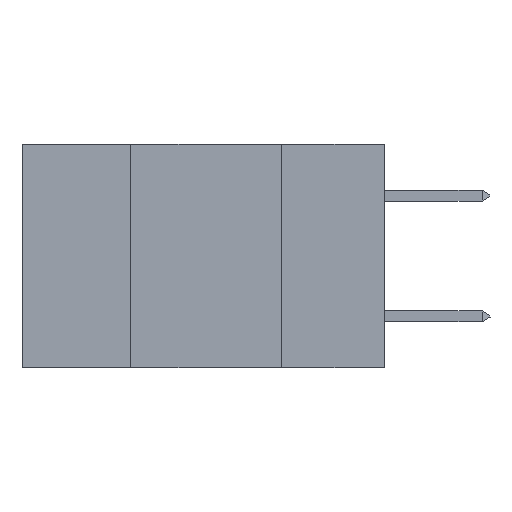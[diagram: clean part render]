
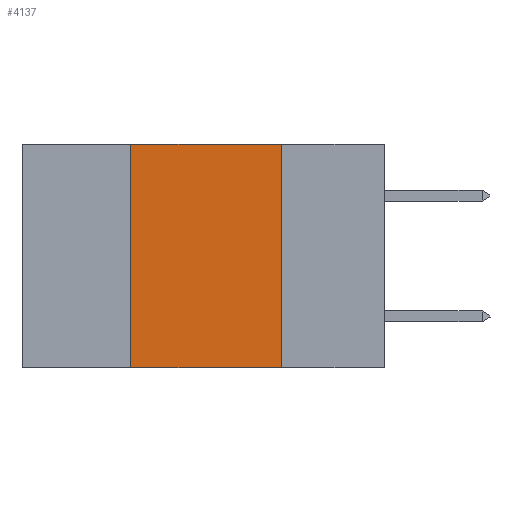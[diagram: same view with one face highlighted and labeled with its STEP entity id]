
A CAD part, left-side view. The second image highlights one B-rep face of the part: STEP entity #4137.
In plain terms, the highlighted planar face has unit normal (-1, 0, 0).
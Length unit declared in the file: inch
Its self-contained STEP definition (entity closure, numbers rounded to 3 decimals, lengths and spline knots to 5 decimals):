
#258 = DIRECTION ( 'NONE',  ( 0., 0., 1. ) ) ;
#322 = ORIENTED_EDGE ( 'NONE', *, *, #5474, .F. ) ;
#654 = CARTESIAN_POINT ( 'NONE',  ( 0., 0.42, 0. ) ) ;
#828 = CARTESIAN_POINT ( 'NONE',  ( 0., 0.17, 0. ) ) ;
#831 = VECTOR ( 'NONE', #3111, 39.37008 ) ;
#1708 = VERTEX_POINT ( 'NONE', #10347 ) ;
#1916 = LINE ( 'NONE', #5691, #11187 ) ;
#2489 = EDGE_CURVE ( 'NONE', #5838, #1708, #4367, .T. ) ;
#2636 = VECTOR ( 'NONE', #7221, 39.37008 ) ;
#3043 = CARTESIAN_POINT ( 'NONE',  ( 0., 0.17, 0. ) ) ;
#3111 = DIRECTION ( 'NONE',  ( 0., -1., 0. ) ) ;
#3341 = VECTOR ( 'NONE', #3395, 39.37008 ) ;
#3395 = DIRECTION ( 'NONE',  ( 0., 0., -1. ) ) ;
#3470 = LINE ( 'NONE', #828, #3341 ) ;
#4081 = ORIENTED_EDGE ( 'NONE', *, *, #5026, .F. ) ;
#4137 = ADVANCED_FACE ( 'NONE', ( #11146 ), #9200, .F. ) ;
#4367 = LINE ( 'NONE', #7265, #2636 ) ;
#4542 = EDGE_CURVE ( 'NONE', #10076, #1708, #3470, .T. ) ;
#4907 = EDGE_LOOP ( 'NONE', ( #11507, #4081, #322, #5097 ) ) ;
#5026 = EDGE_CURVE ( 'NONE', #5121, #10076, #9524, .T. ) ;
#5097 = ORIENTED_EDGE ( 'NONE', *, *, #2489, .T. ) ;
#5121 = VERTEX_POINT ( 'NONE', #654 ) ;
#5474 = EDGE_CURVE ( 'NONE', #5838, #5121, #1916, .T. ) ;
#5507 = CARTESIAN_POINT ( 'NONE',  ( 0., 0.42, -0.37 ) ) ;
#5691 = CARTESIAN_POINT ( 'NONE',  ( 0., 0.42, 0. ) ) ;
#5838 = VERTEX_POINT ( 'NONE', #5507 ) ;
#6012 = DIRECTION ( 'NONE',  ( 1., 0., 0. ) ) ;
#7221 = DIRECTION ( 'NONE',  ( 0., -1., 0. ) ) ;
#7265 = CARTESIAN_POINT ( 'NONE',  ( 0., 0.6, -0.37 ) ) ;
#7489 = CARTESIAN_POINT ( 'NONE',  ( 0., 0.6, 0. ) ) ;
#7505 = DIRECTION ( 'NONE',  ( 0., 0., -1. ) ) ;
#7724 = CARTESIAN_POINT ( 'NONE',  ( 0., 0.6, 0. ) ) ;
#9200 = PLANE ( 'NONE',  #11271 ) ;
#9524 = LINE ( 'NONE', #7724, #831 ) ;
#10076 = VERTEX_POINT ( 'NONE', #3043 ) ;
#10347 = CARTESIAN_POINT ( 'NONE',  ( 0., 0.17, -0.37 ) ) ;
#11146 = FACE_OUTER_BOUND ( 'NONE', #4907, .T. ) ;
#11187 = VECTOR ( 'NONE', #258, 39.37008 ) ;
#11271 = AXIS2_PLACEMENT_3D ( 'NONE', #7489, #6012, #7505 ) ;
#11507 = ORIENTED_EDGE ( 'NONE', *, *, #4542, .F. ) ;
